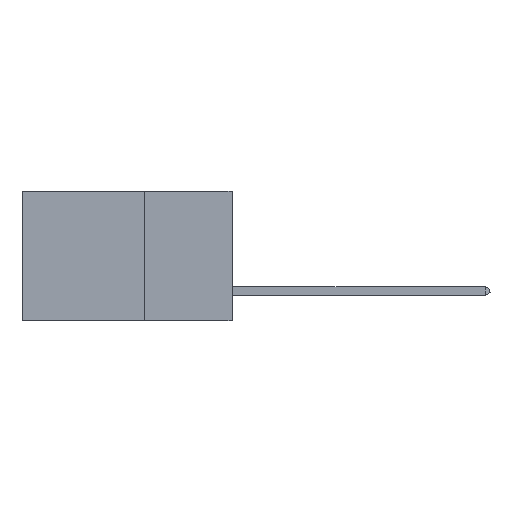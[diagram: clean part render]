
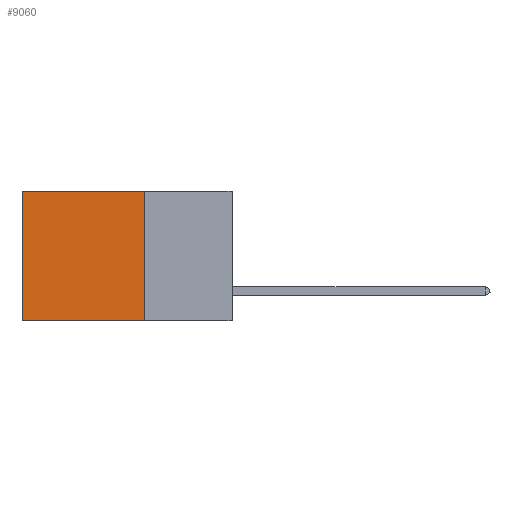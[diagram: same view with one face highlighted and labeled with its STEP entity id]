
A CAD part, left-side view. The second image highlights one B-rep face of the part: STEP entity #9060.
In plain terms, the highlighted planar face has unit normal (-1, 0, 0).
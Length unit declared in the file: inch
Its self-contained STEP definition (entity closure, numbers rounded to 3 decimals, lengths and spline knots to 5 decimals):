
#124 = EDGE_CURVE ( 'NONE', #9804, #233, #12034, .T. ) ;
#233 = VERTEX_POINT ( 'NONE', #6159 ) ;
#478 = AXIS2_PLACEMENT_3D ( 'NONE', #949, #5903, #10878 ) ;
#949 = CARTESIAN_POINT ( 'NONE',  ( 0.2875, 0.25, 0. ) ) ;
#972 = LINE ( 'NONE', #10139, #1162 ) ;
#1162 = VECTOR ( 'NONE', #8719, 39.37008 ) ;
#1618 = CARTESIAN_POINT ( 'NONE',  ( 0.2875, 0.25, -0.37 ) ) ;
#2201 = EDGE_LOOP ( 'NONE', ( #14396, #2718, #4621, #11613 ) ) ;
#2290 = VECTOR ( 'NONE', #15104, 39.37008 ) ;
#2718 = ORIENTED_EDGE ( 'NONE', *, *, #124, .F. ) ;
#3404 = VERTEX_POINT ( 'NONE', #7122 ) ;
#3424 = EDGE_CURVE ( 'NONE', #9713, #3404, #5592, .T. ) ;
#4621 = ORIENTED_EDGE ( 'NONE', *, *, #13768, .F. ) ;
#5552 = CARTESIAN_POINT ( 'NONE',  ( 0.2875, 0.25, 0. ) ) ;
#5592 = LINE ( 'NONE', #14772, #2290 ) ;
#5903 = DIRECTION ( 'NONE',  ( 1., 0., 0. ) ) ;
#6053 = CARTESIAN_POINT ( 'NONE',  ( 0.2875, 0.6, 0. ) ) ;
#6159 = CARTESIAN_POINT ( 'NONE',  ( 0.2875, 0.6, -0.37 ) ) ;
#7042 = LINE ( 'NONE', #6053, #9363 ) ;
#7072 = PLANE ( 'NONE',  #478 ) ;
#7105 = CARTESIAN_POINT ( 'NONE',  ( 0.2875, 0.25, -0.37 ) ) ;
#7122 = CARTESIAN_POINT ( 'NONE',  ( 0.2875, 0.6, 0. ) ) ;
#8414 = DIRECTION ( 'NONE',  ( 0., 0., -1. ) ) ;
#8719 = DIRECTION ( 'NONE',  ( 0., 0., -1. ) ) ;
#9060 = ADVANCED_FACE ( 'NONE', ( #15693 ), #7072, .F. ) ;
#9363 = VECTOR ( 'NONE', #8414, 39.37008 ) ;
#9713 = VERTEX_POINT ( 'NONE', #5552 ) ;
#9804 = VERTEX_POINT ( 'NONE', #7105 ) ;
#10139 = CARTESIAN_POINT ( 'NONE',  ( 0.2875, 0.25, 0. ) ) ;
#10878 = DIRECTION ( 'NONE',  ( 0., 0., -1. ) ) ;
#10879 = VECTOR ( 'NONE', #13955, 39.37008 ) ;
#11613 = ORIENTED_EDGE ( 'NONE', *, *, #3424, .T. ) ;
#12034 = LINE ( 'NONE', #1618, #10879 ) ;
#13768 = EDGE_CURVE ( 'NONE', #9713, #9804, #972, .T. ) ;
#13955 = DIRECTION ( 'NONE',  ( 0., 1., 0. ) ) ;
#14396 = ORIENTED_EDGE ( 'NONE', *, *, #15925, .T. ) ;
#14772 = CARTESIAN_POINT ( 'NONE',  ( 0.2875, 0.25, 0. ) ) ;
#15104 = DIRECTION ( 'NONE',  ( 0., 1., 0. ) ) ;
#15693 = FACE_OUTER_BOUND ( 'NONE', #2201, .T. ) ;
#15925 = EDGE_CURVE ( 'NONE', #3404, #233, #7042, .T. ) ;
